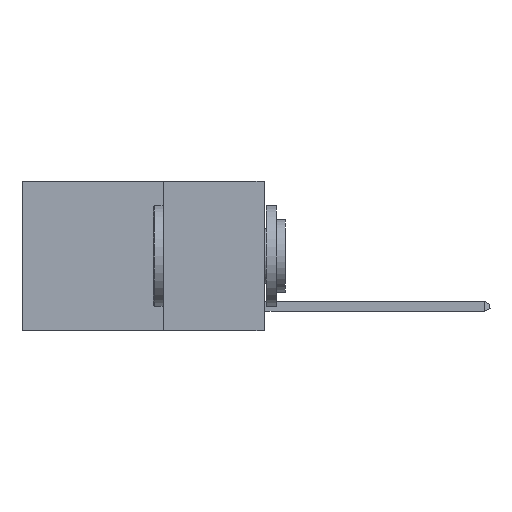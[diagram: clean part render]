
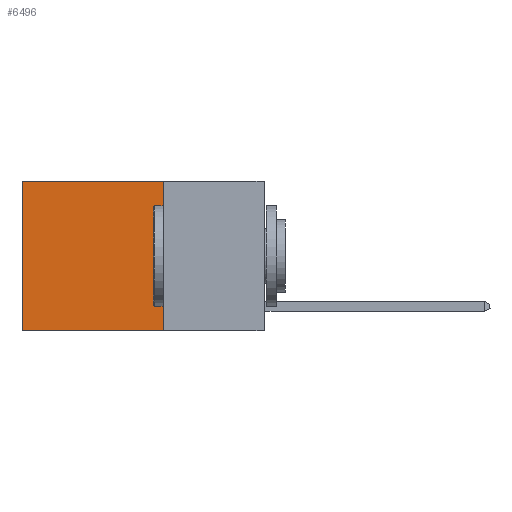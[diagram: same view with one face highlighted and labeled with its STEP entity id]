
A CAD part, left-side view. The second image highlights one B-rep face of the part: STEP entity #6496.
In plain terms, the highlighted planar face has unit normal (-1, 0, 0).
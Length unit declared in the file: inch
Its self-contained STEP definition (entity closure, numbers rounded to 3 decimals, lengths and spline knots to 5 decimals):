
#1126 = CARTESIAN_POINT ( 'NONE',  ( 0.2625, 0.6, 0. ) ) ;
#1561 = CARTESIAN_POINT ( 'NONE',  ( 0.2625, 0.25, 0. ) ) ;
#1992 = EDGE_CURVE ( 'NONE', #13147, #22730, #14295, .T. ) ;
#2258 = DIRECTION ( 'NONE',  ( 1., 0., 0. ) ) ;
#3400 = LINE ( 'NONE', #1561, #4354 ) ;
#3778 = CARTESIAN_POINT ( 'NONE',  ( 0.2625, 0.25, 0. ) ) ;
#3852 = CARTESIAN_POINT ( 'NONE',  ( 0.2625, 0.25, 0. ) ) ;
#4091 = AXIS2_PLACEMENT_3D ( 'NONE', #3852, #2258, #8163 ) ;
#4184 = CARTESIAN_POINT ( 'NONE',  ( 0.2625, 0.6, 0. ) ) ;
#4354 = VECTOR ( 'NONE', #19045, 39.37008 ) ;
#4679 = EDGE_LOOP ( 'NONE', ( #18149, #25161, #20047, #23699 ) ) ;
#6496 = ADVANCED_FACE ( 'NONE', ( #13781 ), #15983, .F. ) ;
#8163 = DIRECTION ( 'NONE',  ( 0., 0., -1. ) ) ;
#8726 = EDGE_CURVE ( 'NONE', #22005, #22730, #14117, .T. ) ;
#9680 = VECTOR ( 'NONE', #22741, 39.37008 ) ;
#12146 = DIRECTION ( 'NONE',  ( 0., 0., -1. ) ) ;
#12532 = LINE ( 'NONE', #18262, #16517 ) ;
#13147 = VERTEX_POINT ( 'NONE', #24095 ) ;
#13781 = FACE_OUTER_BOUND ( 'NONE', #4679, .T. ) ;
#14117 = LINE ( 'NONE', #4184, #18682 ) ;
#14223 = VERTEX_POINT ( 'NONE', #3778 ) ;
#14295 = LINE ( 'NONE', #18698, #9680 ) ;
#15983 = PLANE ( 'NONE',  #4091 ) ;
#16517 = VECTOR ( 'NONE', #22297, 39.37008 ) ;
#18149 = ORIENTED_EDGE ( 'NONE', *, *, #8726, .T. ) ;
#18262 = CARTESIAN_POINT ( 'NONE',  ( 0.2625, 0.25, 0. ) ) ;
#18682 = VECTOR ( 'NONE', #12146, 39.37008 ) ;
#18698 = CARTESIAN_POINT ( 'NONE',  ( 0.2625, 0.25, -0.37 ) ) ;
#19045 = DIRECTION ( 'NONE',  ( 0., 0., -1. ) ) ;
#19838 = CARTESIAN_POINT ( 'NONE',  ( 0.2625, 0.6, -0.37 ) ) ;
#20047 = ORIENTED_EDGE ( 'NONE', *, *, #22980, .F. ) ;
#21755 = EDGE_CURVE ( 'NONE', #14223, #22005, #12532, .T. ) ;
#22005 = VERTEX_POINT ( 'NONE', #1126 ) ;
#22297 = DIRECTION ( 'NONE',  ( 0., 1., 0. ) ) ;
#22730 = VERTEX_POINT ( 'NONE', #19838 ) ;
#22741 = DIRECTION ( 'NONE',  ( 0., 1., 0. ) ) ;
#22980 = EDGE_CURVE ( 'NONE', #14223, #13147, #3400, .T. ) ;
#23699 = ORIENTED_EDGE ( 'NONE', *, *, #21755, .T. ) ;
#24095 = CARTESIAN_POINT ( 'NONE',  ( 0.2625, 0.25, -0.37 ) ) ;
#25161 = ORIENTED_EDGE ( 'NONE', *, *, #1992, .F. ) ;
